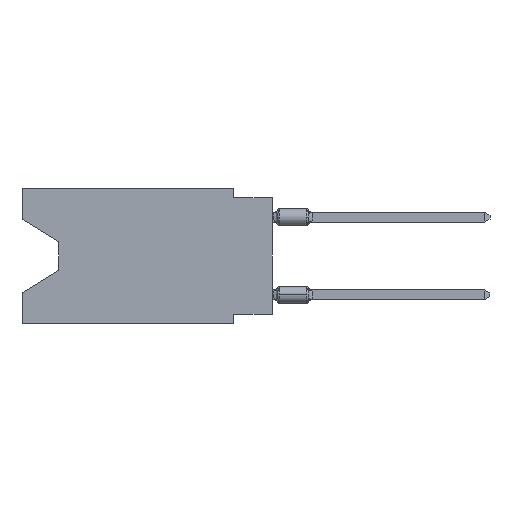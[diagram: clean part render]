
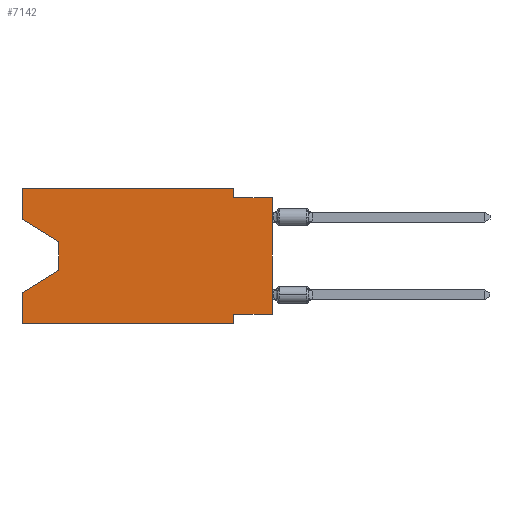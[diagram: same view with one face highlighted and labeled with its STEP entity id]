
A CAD part, left-side view. The second image highlights one B-rep face of the part: STEP entity #7142.
In plain terms, the highlighted planar face has unit normal (-1, 0, 0).
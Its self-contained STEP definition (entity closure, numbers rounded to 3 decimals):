
#150 = DIRECTION ( 'NONE',  ( 0., -1., 0. ) ) ;
#306 = DIRECTION ( 'NONE',  ( 0., 0., 1. ) ) ;
#458 = DIRECTION ( 'NONE',  ( 0., 0., -1. ) ) ;
#506 = VERTEX_POINT ( 'NONE', #6308 ) ;
#716 = CARTESIAN_POINT ( 'NONE',  ( 0., 13.97, -5.385 ) ) ;
#785 = CARTESIAN_POINT ( 'NONE',  ( 0., 16.383, 0. ) ) ;
#831 = AXIS2_PLACEMENT_3D ( 'NONE', #785, #13412, #3953 ) ;
#917 = DIRECTION ( 'NONE',  ( 0., 0., -1. ) ) ;
#949 = VERTEX_POINT ( 'NONE', #1041 ) ;
#1017 = VECTOR ( 'NONE', #11416, 1000. ) ;
#1041 = CARTESIAN_POINT ( 'NONE',  ( 0., 16.383, -6.852 ) ) ;
#1172 = CARTESIAN_POINT ( 'NONE',  ( 0., 2.54, 0. ) ) ;
#1186 = LINE ( 'NONE', #5401, #4733 ) ;
#1209 = ORIENTED_EDGE ( 'NONE', *, *, #4765, .F. ) ;
#1240 = DIRECTION ( 'NONE',  ( 0., -0.855, -0.519 ) ) ;
#1497 = LINE ( 'NONE', #9914, #3039 ) ;
#1516 = LINE ( 'NONE', #8068, #10770 ) ;
#1731 = CARTESIAN_POINT ( 'NONE',  ( 0., 0., -8.255 ) ) ;
#1918 = VECTOR ( 'NONE', #917, 1000. ) ;
#1953 = CARTESIAN_POINT ( 'NONE',  ( 0., 2.54, -8.89 ) ) ;
#2232 = EDGE_CURVE ( 'NONE', #506, #7207, #8764, .T. ) ;
#2283 = VERTEX_POINT ( 'NONE', #1172 ) ;
#2499 = CARTESIAN_POINT ( 'NONE',  ( 0., 16.383, 0. ) ) ;
#2850 = VECTOR ( 'NONE', #4215, 1000. ) ;
#3039 = VECTOR ( 'NONE', #458, 1000. ) ;
#3241 = VECTOR ( 'NONE', #11320, 1000. ) ;
#3273 = LINE ( 'NONE', #9421, #13344 ) ;
#3523 = DIRECTION ( 'NONE',  ( 0., 0., 1. ) ) ;
#3595 = LINE ( 'NONE', #2499, #10344 ) ;
#3710 = VERTEX_POINT ( 'NONE', #1731 ) ;
#3953 = DIRECTION ( 'NONE',  ( 0., 0., -1. ) ) ;
#4024 = CARTESIAN_POINT ( 'NONE',  ( 0., 2.54, -8.89 ) ) ;
#4142 = VERTEX_POINT ( 'NONE', #5779 ) ;
#4215 = DIRECTION ( 'NONE',  ( 0., 0., -1. ) ) ;
#4315 = EDGE_CURVE ( 'NONE', #12097, #2283, #13494, .T. ) ;
#4541 = CARTESIAN_POINT ( 'NONE',  ( 0., 16.383, -2.038 ) ) ;
#4627 = VERTEX_POINT ( 'NONE', #716 ) ;
#4649 = ORIENTED_EDGE ( 'NONE', *, *, #2232, .T. ) ;
#4733 = VECTOR ( 'NONE', #150, 1000. ) ;
#4765 = EDGE_CURVE ( 'NONE', #6910, #7207, #7200, .T. ) ;
#5401 = CARTESIAN_POINT ( 'NONE',  ( 0., 0., -0.635 ) ) ;
#5779 = CARTESIAN_POINT ( 'NONE',  ( 0., 13.97, -3.505 ) ) ;
#6031 = PLANE ( 'NONE',  #831 ) ;
#6171 = ORIENTED_EDGE ( 'NONE', *, *, #10513, .F. ) ;
#6308 = CARTESIAN_POINT ( 'NONE',  ( 0., 16.383, -8.89 ) ) ;
#6516 = CARTESIAN_POINT ( 'NONE',  ( 0., 16.383, 0. ) ) ;
#6664 = CARTESIAN_POINT ( 'NONE',  ( 0., 0., -0.635 ) ) ;
#6685 = EDGE_CURVE ( 'NONE', #4627, #949, #1516, .T. ) ;
#6766 = VERTEX_POINT ( 'NONE', #8203 ) ;
#6901 = ORIENTED_EDGE ( 'NONE', *, *, #4315, .F. ) ;
#6910 = VERTEX_POINT ( 'NONE', #7645 ) ;
#7142 = ADVANCED_FACE ( 'NONE', ( #13098 ), #6031, .F. ) ;
#7200 = LINE ( 'NONE', #1953, #1918 ) ;
#7207 = VERTEX_POINT ( 'NONE', #4024 ) ;
#7376 = EDGE_CURVE ( 'NONE', #506, #949, #3595, .T. ) ;
#7427 = ORIENTED_EDGE ( 'NONE', *, *, #8121, .T. ) ;
#7440 = EDGE_CURVE ( 'NONE', #3710, #6910, #9118, .T. ) ;
#7645 = CARTESIAN_POINT ( 'NONE',  ( 0., 2.54, -8.255 ) ) ;
#8068 = CARTESIAN_POINT ( 'NONE',  ( 0., 13.97, -5.385 ) ) ;
#8121 = EDGE_CURVE ( 'NONE', #4142, #4627, #1497, .T. ) ;
#8140 = EDGE_CURVE ( 'NONE', #9722, #4142, #11787, .T. ) ;
#8203 = CARTESIAN_POINT ( 'NONE',  ( 0., 2.54, -0.635 ) ) ;
#8418 = ORIENTED_EDGE ( 'NONE', *, *, #7376, .F. ) ;
#8636 = EDGE_LOOP ( 'NONE', ( #11377, #7427, #10556, #8418, #4649, #1209, #10530, #11848, #6171, #13537, #6901, #10944 ) ) ;
#8764 = LINE ( 'NONE', #10832, #10654 ) ;
#9118 = LINE ( 'NONE', #12082, #3241 ) ;
#9275 = VECTOR ( 'NONE', #306, 1000. ) ;
#9421 = CARTESIAN_POINT ( 'NONE',  ( 0., 0., 0. ) ) ;
#9652 = VECTOR ( 'NONE', #1240, 1000. ) ;
#9722 = VERTEX_POINT ( 'NONE', #4541 ) ;
#9914 = CARTESIAN_POINT ( 'NONE',  ( 0., 13.97, -3.505 ) ) ;
#9933 = CARTESIAN_POINT ( 'NONE',  ( 0., 16.383, -2.038 ) ) ;
#10344 = VECTOR ( 'NONE', #3523, 1000. ) ;
#10513 = EDGE_CURVE ( 'NONE', #6766, #11308, #1186, .T. ) ;
#10530 = ORIENTED_EDGE ( 'NONE', *, *, #7440, .F. ) ;
#10556 = ORIENTED_EDGE ( 'NONE', *, *, #6685, .T. ) ;
#10654 = VECTOR ( 'NONE', #10692, 1000. ) ;
#10692 = DIRECTION ( 'NONE',  ( 0., -1., 0. ) ) ;
#10770 = VECTOR ( 'NONE', #10962, 1000. ) ;
#10832 = CARTESIAN_POINT ( 'NONE',  ( 0., 16.383, -8.89 ) ) ;
#10944 = ORIENTED_EDGE ( 'NONE', *, *, #13146, .F. ) ;
#10962 = DIRECTION ( 'NONE',  ( 0., 0.855, -0.519 ) ) ;
#11231 = EDGE_CURVE ( 'NONE', #3710, #11308, #3273, .T. ) ;
#11308 = VERTEX_POINT ( 'NONE', #6664 ) ;
#11320 = DIRECTION ( 'NONE',  ( 0., 1., 0. ) ) ;
#11377 = ORIENTED_EDGE ( 'NONE', *, *, #8140, .T. ) ;
#11416 = DIRECTION ( 'NONE',  ( 0., -1., 0. ) ) ;
#11787 = LINE ( 'NONE', #9933, #9652 ) ;
#11825 = LINE ( 'NONE', #6516, #9275 ) ;
#11848 = ORIENTED_EDGE ( 'NONE', *, *, #11231, .T. ) ;
#12082 = CARTESIAN_POINT ( 'NONE',  ( 0., 0., -8.255 ) ) ;
#12097 = VERTEX_POINT ( 'NONE', #12871 ) ;
#12518 = EDGE_CURVE ( 'NONE', #2283, #6766, #12781, .T. ) ;
#12525 = CARTESIAN_POINT ( 'NONE',  ( 0., 16.383, 0. ) ) ;
#12574 = CARTESIAN_POINT ( 'NONE',  ( 0., 2.54, 0. ) ) ;
#12781 = LINE ( 'NONE', #12574, #2850 ) ;
#12871 = CARTESIAN_POINT ( 'NONE',  ( 0., 16.383, 0. ) ) ;
#13098 = FACE_OUTER_BOUND ( 'NONE', #8636, .T. ) ;
#13146 = EDGE_CURVE ( 'NONE', #9722, #12097, #11825, .T. ) ;
#13344 = VECTOR ( 'NONE', #13636, 1000. ) ;
#13412 = DIRECTION ( 'NONE',  ( 1., 0., 0. ) ) ;
#13494 = LINE ( 'NONE', #12525, #1017 ) ;
#13537 = ORIENTED_EDGE ( 'NONE', *, *, #12518, .F. ) ;
#13636 = DIRECTION ( 'NONE',  ( 0., 0., 1. ) ) ;
